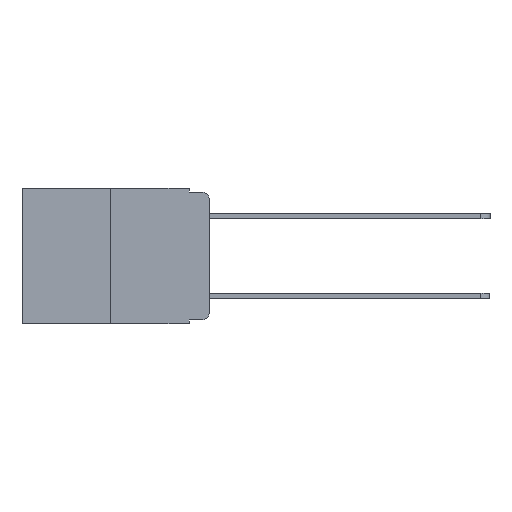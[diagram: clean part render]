
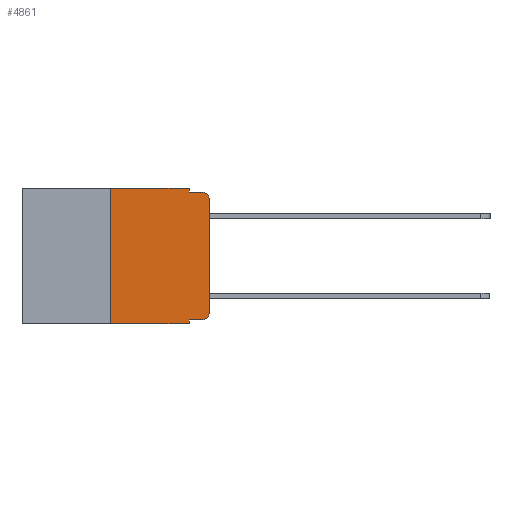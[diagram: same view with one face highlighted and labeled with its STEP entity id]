
A CAD part, left-side view. The second image highlights one B-rep face of the part: STEP entity #4861.
In plain terms, the highlighted planar face has unit normal (-1, 0, 0).
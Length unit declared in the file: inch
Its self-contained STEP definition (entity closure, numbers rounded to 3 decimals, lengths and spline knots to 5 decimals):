
#179 = ORIENTED_EDGE ( 'NONE', *, *, #234, .F. ) ;
#234 = EDGE_CURVE ( 'NONE', #6652, #1650, #7297, .T. ) ;
#274 = FACE_OUTER_BOUND ( 'NONE', #5251, .T. ) ;
#325 = AXIS2_PLACEMENT_3D ( 'NONE', #11850, #6200, #12755 ) ;
#372 = ORIENTED_EDGE ( 'NONE', *, *, #12443, .F. ) ;
#392 = ORIENTED_EDGE ( 'NONE', *, *, #9059, .T. ) ;
#406 = ORIENTED_EDGE ( 'NONE', *, *, #8726, .F. ) ;
#444 = VERTEX_POINT ( 'NONE', #5204 ) ;
#579 = ORIENTED_EDGE ( 'NONE', *, *, #8080, .T. ) ;
#628 = DIRECTION ( 'NONE',  ( 0., 0., 1. ) ) ;
#682 = ORIENTED_EDGE ( 'NONE', *, *, #7448, .T. ) ;
#1013 = EDGE_CURVE ( 'NONE', #6925, #1650, #1033, .T. ) ;
#1016 = CARTESIAN_POINT ( 'NONE',  ( 0., 0.051, -0.333 ) ) ;
#1033 = CIRCLE ( 'NONE', #1732, 0.02 ) ;
#1045 = DIRECTION ( 'NONE',  ( 0., 0., -1. ) ) ;
#1418 = CIRCLE ( 'NONE', #325, 0.02 ) ;
#1552 = VECTOR ( 'NONE', #5156, 39.37008 ) ;
#1650 = VERTEX_POINT ( 'NONE', #7419 ) ;
#1711 = EDGE_CURVE ( 'NONE', #5960, #6925, #12096, .T. ) ;
#1732 = AXIS2_PLACEMENT_3D ( 'NONE', #12296, #5350, #12169 ) ;
#2123 = VERTEX_POINT ( 'NONE', #10420 ) ;
#2413 = CARTESIAN_POINT ( 'NONE',  ( 0., 0.473, 0. ) ) ;
#2461 = CARTESIAN_POINT ( 'NONE',  ( 0., 0.051, 0. ) ) ;
#3197 = CARTESIAN_POINT ( 'NONE',  ( 0., 0.051, -0.333 ) ) ;
#3282 = DIRECTION ( 'NONE',  ( 0., -1., 0. ) ) ;
#3366 = LINE ( 'NONE', #6413, #7955 ) ;
#3720 = CARTESIAN_POINT ( 'NONE',  ( 0., 0.051, -0.343 ) ) ;
#3784 = EDGE_CURVE ( 'NONE', #444, #2123, #10841, .T. ) ;
#4157 = CARTESIAN_POINT ( 'NONE',  ( 0., 0.051, -0.01 ) ) ;
#4506 = VECTOR ( 'NONE', #628, 39.37008 ) ;
#4580 = VERTEX_POINT ( 'NONE', #3720 ) ;
#4861 = ADVANCED_FACE ( 'NONE', ( #274 ), #7746, .F. ) ;
#5027 = ORIENTED_EDGE ( 'NONE', *, *, #3784, .F. ) ;
#5091 = ORIENTED_EDGE ( 'NONE', *, *, #11243, .F. ) ;
#5156 = DIRECTION ( 'NONE',  ( 0., -1., 0. ) ) ;
#5204 = CARTESIAN_POINT ( 'NONE',  ( 0., 0.25, 0. ) ) ;
#5251 = EDGE_LOOP ( 'NONE', ( #7211, #7851, #179, #372, #5027, #5091, #392, #406, #579, #682 ) ) ;
#5350 = DIRECTION ( 'NONE',  ( -1., 0., 0. ) ) ;
#5744 = VECTOR ( 'NONE', #7038, 39.37008 ) ;
#5960 = VERTEX_POINT ( 'NONE', #12464 ) ;
#6049 = LINE ( 'NONE', #9867, #5744 ) ;
#6200 = DIRECTION ( 'NONE',  ( -1., 0., 0. ) ) ;
#6274 = DIRECTION ( 'NONE',  ( 0., 0., -1. ) ) ;
#6286 = DIRECTION ( 'NONE',  ( 1., 0., 0. ) ) ;
#6413 = CARTESIAN_POINT ( 'NONE',  ( 0., 0.25, 0. ) ) ;
#6652 = VERTEX_POINT ( 'NONE', #4157 ) ;
#6916 = CARTESIAN_POINT ( 'NONE',  ( 0., 0., 0. ) ) ;
#6925 = VERTEX_POINT ( 'NONE', #8336 ) ;
#6967 = LINE ( 'NONE', #2461, #11654 ) ;
#7038 = DIRECTION ( 'NONE',  ( 0., -1., 0. ) ) ;
#7116 = VERTEX_POINT ( 'NONE', #8445 ) ;
#7192 = VECTOR ( 'NONE', #1045, 39.37008 ) ;
#7211 = ORIENTED_EDGE ( 'NONE', *, *, #1711, .T. ) ;
#7297 = LINE ( 'NONE', #10382, #9251 ) ;
#7378 = DIRECTION ( 'NONE',  ( 0., 0., 1. ) ) ;
#7419 = CARTESIAN_POINT ( 'NONE',  ( 0., 0.02, -0.01 ) ) ;
#7448 = EDGE_CURVE ( 'NONE', #8562, #5960, #1418, .T. ) ;
#7733 = CARTESIAN_POINT ( 'NONE',  ( 0., 0.473, 0. ) ) ;
#7746 = PLANE ( 'NONE',  #9178 ) ;
#7851 = ORIENTED_EDGE ( 'NONE', *, *, #1013, .T. ) ;
#7955 = VECTOR ( 'NONE', #7378, 39.37008 ) ;
#8080 = EDGE_CURVE ( 'NONE', #8538, #8562, #9556, .T. ) ;
#8139 = CARTESIAN_POINT ( 'NONE',  ( 0., 0.051, 0. ) ) ;
#8336 = CARTESIAN_POINT ( 'NONE',  ( 0., 0., -0.03 ) ) ;
#8411 = DIRECTION ( 'NONE',  ( 0., 0., -1. ) ) ;
#8445 = CARTESIAN_POINT ( 'NONE',  ( 0., 0.25, -0.343 ) ) ;
#8538 = VERTEX_POINT ( 'NONE', #1016 ) ;
#8562 = VERTEX_POINT ( 'NONE', #12768 ) ;
#8726 = EDGE_CURVE ( 'NONE', #8538, #4580, #6967, .T. ) ;
#8903 = DIRECTION ( 'NONE',  ( 0., -1., 0. ) ) ;
#9059 = EDGE_CURVE ( 'NONE', #7116, #4580, #6049, .T. ) ;
#9178 = AXIS2_PLACEMENT_3D ( 'NONE', #7733, #6286, #6274 ) ;
#9251 = VECTOR ( 'NONE', #8903, 39.37008 ) ;
#9556 = LINE ( 'NONE', #3197, #1552 ) ;
#9724 = LINE ( 'NONE', #8139, #7192 ) ;
#9867 = CARTESIAN_POINT ( 'NONE',  ( 0., 0.473, -0.343 ) ) ;
#10382 = CARTESIAN_POINT ( 'NONE',  ( 0., 0.051, -0.01 ) ) ;
#10420 = CARTESIAN_POINT ( 'NONE',  ( 0., 0.051, 0. ) ) ;
#10841 = LINE ( 'NONE', #2413, #11418 ) ;
#11243 = EDGE_CURVE ( 'NONE', #7116, #444, #3366, .T. ) ;
#11418 = VECTOR ( 'NONE', #3282, 39.37008 ) ;
#11654 = VECTOR ( 'NONE', #8411, 39.37008 ) ;
#11850 = CARTESIAN_POINT ( 'NONE',  ( 0., 0.02, -0.313 ) ) ;
#12096 = LINE ( 'NONE', #6916, #4506 ) ;
#12169 = DIRECTION ( 'NONE',  ( 0., 0., -1. ) ) ;
#12296 = CARTESIAN_POINT ( 'NONE',  ( 0., 0.02, -0.03 ) ) ;
#12443 = EDGE_CURVE ( 'NONE', #2123, #6652, #9724, .T. ) ;
#12464 = CARTESIAN_POINT ( 'NONE',  ( 0., 0., -0.313 ) ) ;
#12755 = DIRECTION ( 'NONE',  ( 0., 0., -1. ) ) ;
#12768 = CARTESIAN_POINT ( 'NONE',  ( 0., 0.02, -0.333 ) ) ;
